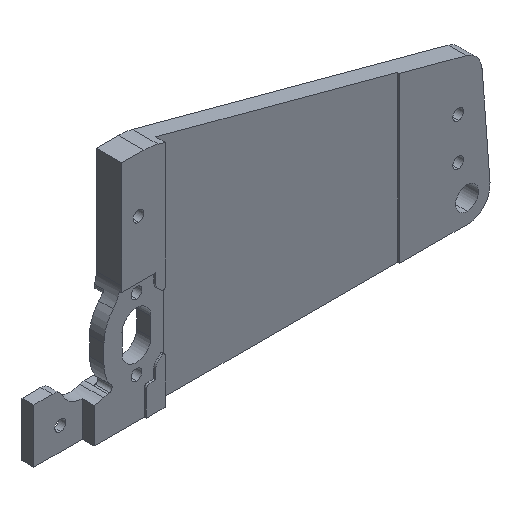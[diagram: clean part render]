
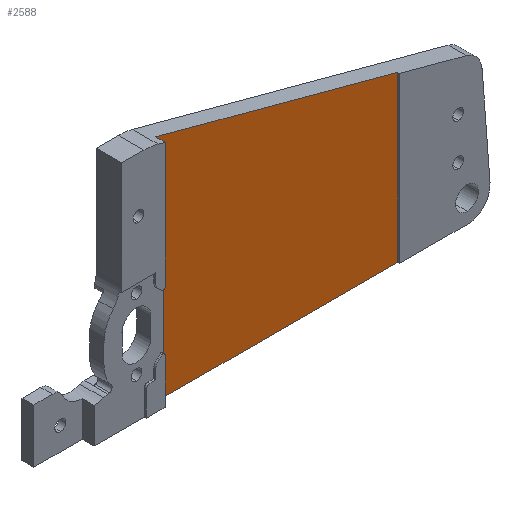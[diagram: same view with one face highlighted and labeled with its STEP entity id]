
A CAD part, isometric view. The second image highlights one B-rep face of the part: STEP entity #2588.
In plain terms, the highlighted planar face has unit normal (0, -1, 0).
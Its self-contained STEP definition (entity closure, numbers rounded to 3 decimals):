
#504 = LINE ( 'NONE', #2440, #884 ) ;
#737 = AXIS2_PLACEMENT_3D ( 'NONE', #2191, #1927, #3310 ) ;
#785 = DIRECTION ( 'NONE',  ( 0., 0., -1. ) ) ;
#790 = EDGE_CURVE ( 'NONE', #802, #1373, #1449, .T. ) ;
#802 = VERTEX_POINT ( 'NONE', #1802 ) ;
#871 = CARTESIAN_POINT ( 'NONE',  ( 10.432, 2.545, 0. ) ) ;
#884 = VECTOR ( 'NONE', #2179, 1000. ) ;
#922 = CARTESIAN_POINT ( 'NONE',  ( 77.132, 2.545, -18.971 ) ) ;
#978 = EDGE_CURVE ( 'NONE', #1373, #1350, #2413, .T. ) ;
#1044 = LINE ( 'NONE', #3208, #1924 ) ;
#1149 = PLANE ( 'NONE',  #737 ) ;
#1350 = VERTEX_POINT ( 'NONE', #2331 ) ;
#1373 = VERTEX_POINT ( 'NONE', #1491 ) ;
#1449 = LINE ( 'NONE', #871, #2923 ) ;
#1491 = CARTESIAN_POINT ( 'NONE',  ( 10.432, 2.545, -64.364 ) ) ;
#1719 = FACE_OUTER_BOUND ( 'NONE', #2364, .T. ) ;
#1802 = CARTESIAN_POINT ( 'NONE',  ( 10.432, 2.545, -1.036 ) ) ;
#1924 = VECTOR ( 'NONE', #785, 1000. ) ;
#1927 = DIRECTION ( 'NONE',  ( 0., -1., 0. ) ) ;
#1973 = DIRECTION ( 'NONE',  ( 1., 0., 0. ) ) ;
#2065 = DIRECTION ( 'NONE',  ( 0., 0., -1. ) ) ;
#2166 = EDGE_CURVE ( 'NONE', #2776, #802, #504, .T. ) ;
#2179 = DIRECTION ( 'NONE',  ( -0.966, 0., 0.26 ) ) ;
#2191 = CARTESIAN_POINT ( 'NONE',  ( 0., 2.545, 0. ) ) ;
#2246 = VECTOR ( 'NONE', #1973, 1000. ) ;
#2331 = CARTESIAN_POINT ( 'NONE',  ( 77.132, 2.545, -64.364 ) ) ;
#2364 = EDGE_LOOP ( 'NONE', ( #2767, #3286, #2846, #3346 ) ) ;
#2413 = LINE ( 'NONE', #2899, #2246 ) ;
#2440 = CARTESIAN_POINT ( 'NONE',  ( 78.632, 2.545, -19.375 ) ) ;
#2588 = ADVANCED_FACE ( 'NONE', ( #1719 ), #1149, .T. ) ;
#2767 = ORIENTED_EDGE ( 'NONE', *, *, #3265, .F. ) ;
#2776 = VERTEX_POINT ( 'NONE', #922 ) ;
#2846 = ORIENTED_EDGE ( 'NONE', *, *, #790, .T. ) ;
#2899 = CARTESIAN_POINT ( 'NONE',  ( 11.932, 2.545, -64.364 ) ) ;
#2923 = VECTOR ( 'NONE', #2065, 1000. ) ;
#3208 = CARTESIAN_POINT ( 'NONE',  ( 77.132, 2.545, -17.55 ) ) ;
#3265 = EDGE_CURVE ( 'NONE', #2776, #1350, #1044, .T. ) ;
#3286 = ORIENTED_EDGE ( 'NONE', *, *, #2166, .T. ) ;
#3310 = DIRECTION ( 'NONE',  ( 1., 0., 0. ) ) ;
#3346 = ORIENTED_EDGE ( 'NONE', *, *, #978, .T. ) ;
